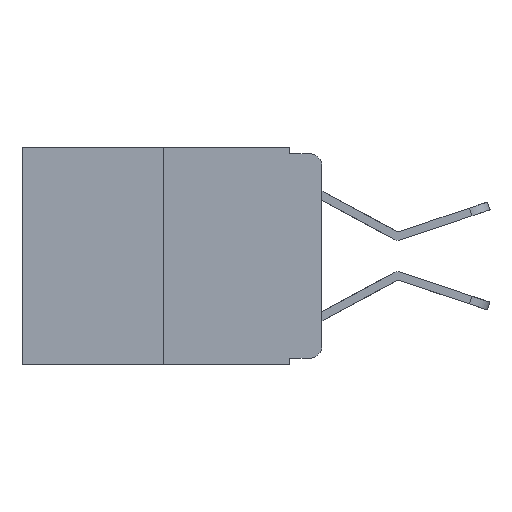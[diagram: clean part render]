
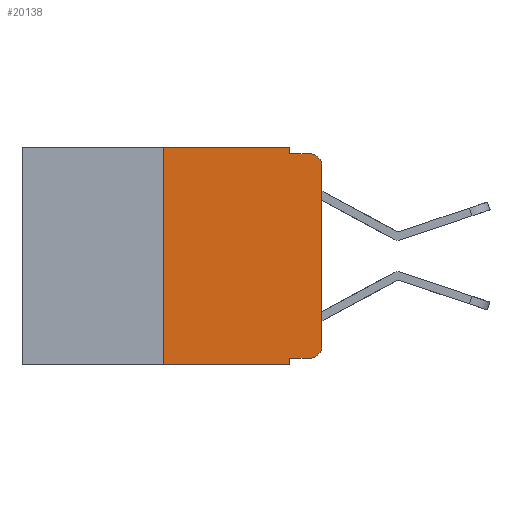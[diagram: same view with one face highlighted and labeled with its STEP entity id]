
A CAD part, left-side view. The second image highlights one B-rep face of the part: STEP entity #20138.
In plain terms, the highlighted planar face has unit normal (-1, 0, 0).
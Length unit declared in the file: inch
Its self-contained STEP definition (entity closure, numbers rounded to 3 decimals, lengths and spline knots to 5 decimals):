
#455 = ORIENTED_EDGE ( 'NONE', *, *, #19903, .F. ) ;
#567 = VERTEX_POINT ( 'NONE', #24018 ) ;
#948 = CARTESIAN_POINT ( 'NONE',  ( 0., 0.25, 0. ) ) ;
#1726 = EDGE_CURVE ( 'NONE', #22850, #15230, #16019, .T. ) ;
#1812 = ORIENTED_EDGE ( 'NONE', *, *, #18586, .F. ) ;
#2081 = DIRECTION ( 'NONE',  ( 0., -1., 0. ) ) ;
#2087 = CARTESIAN_POINT ( 'NONE',  ( 0., 0.473, -0.343 ) ) ;
#2371 = CARTESIAN_POINT ( 'NONE',  ( 0., 0.051, -0.333 ) ) ;
#2601 = CIRCLE ( 'NONE', #25285, 0.02 ) ;
#2778 = CARTESIAN_POINT ( 'NONE',  ( 0., 0.02, -0.03 ) ) ;
#3517 = VECTOR ( 'NONE', #15218, 39.37008 ) ;
#3931 = CARTESIAN_POINT ( 'NONE',  ( 0., 0.473, 0. ) ) ;
#3943 = VECTOR ( 'NONE', #12380, 39.37008 ) ;
#4050 = CARTESIAN_POINT ( 'NONE',  ( 0., 0., -0.03 ) ) ;
#4068 = DIRECTION ( 'NONE',  ( 0., 0., -1. ) ) ;
#4159 = CIRCLE ( 'NONE', #19298, 0.02 ) ;
#4498 = CARTESIAN_POINT ( 'NONE',  ( 0., 0.051, 0. ) ) ;
#4652 = VERTEX_POINT ( 'NONE', #20913 ) ;
#4718 = CARTESIAN_POINT ( 'NONE',  ( 0., 0.051, -0.01 ) ) ;
#4933 = DIRECTION ( 'NONE',  ( 0., 0., -1. ) ) ;
#5468 = CARTESIAN_POINT ( 'NONE',  ( 0., 0.02, -0.01 ) ) ;
#6043 = DIRECTION ( 'NONE',  ( 0., 0., -1. ) ) ;
#6122 = ORIENTED_EDGE ( 'NONE', *, *, #9613, .T. ) ;
#6230 = VERTEX_POINT ( 'NONE', #2371 ) ;
#7003 = VERTEX_POINT ( 'NONE', #11039 ) ;
#7270 = CARTESIAN_POINT ( 'NONE',  ( 0., 0.051, -0.01 ) ) ;
#7398 = ORIENTED_EDGE ( 'NONE', *, *, #17284, .T. ) ;
#7729 = VECTOR ( 'NONE', #18364, 39.37008 ) ;
#7857 = LINE ( 'NONE', #17208, #17907 ) ;
#8035 = CARTESIAN_POINT ( 'NONE',  ( 0., 0.02, -0.313 ) ) ;
#8045 = ORIENTED_EDGE ( 'NONE', *, *, #14597, .T. ) ;
#8287 = CARTESIAN_POINT ( 'NONE',  ( 0., 0.25, 0. ) ) ;
#8868 = LINE ( 'NONE', #18357, #19197 ) ;
#8964 = DIRECTION ( 'NONE',  ( 0., -1., 0. ) ) ;
#9008 = ORIENTED_EDGE ( 'NONE', *, *, #1726, .T. ) ;
#9306 = CARTESIAN_POINT ( 'NONE',  ( 0., 0., -0.313 ) ) ;
#9437 = LINE ( 'NONE', #15255, #25722 ) ;
#9613 = EDGE_CURVE ( 'NONE', #4652, #567, #13111, .T. ) ;
#9634 = VECTOR ( 'NONE', #4068, 39.37008 ) ;
#10115 = DIRECTION ( 'NONE',  ( 0., 0., -1. ) ) ;
#10415 = AXIS2_PLACEMENT_3D ( 'NONE', #3931, #18091, #6043 ) ;
#11039 = CARTESIAN_POINT ( 'NONE',  ( 0., 0.02, -0.333 ) ) ;
#12074 = PLANE ( 'NONE',  #10415 ) ;
#12380 = DIRECTION ( 'NONE',  ( 0., 0., 1. ) ) ;
#12820 = FACE_OUTER_BOUND ( 'NONE', #22519, .T. ) ;
#13111 = LINE ( 'NONE', #2087, #7729 ) ;
#13141 = LINE ( 'NONE', #948, #3517 ) ;
#14327 = ORIENTED_EDGE ( 'NONE', *, *, #25070, .T. ) ;
#14597 = EDGE_CURVE ( 'NONE', #7003, #22850, #4159, .T. ) ;
#15195 = DIRECTION ( 'NONE',  ( 0., 0., -1. ) ) ;
#15218 = DIRECTION ( 'NONE',  ( 0., 0., 1. ) ) ;
#15230 = VERTEX_POINT ( 'NONE', #4050 ) ;
#15255 = CARTESIAN_POINT ( 'NONE',  ( 0., 0.473, 0. ) ) ;
#16019 = LINE ( 'NONE', #22169, #3943 ) ;
#16214 = ORIENTED_EDGE ( 'NONE', *, *, #19267, .F. ) ;
#16226 = CARTESIAN_POINT ( 'NONE',  ( 0., 0.051, 0. ) ) ;
#17026 = DIRECTION ( 'NONE',  ( -1., 0., 0. ) ) ;
#17208 = CARTESIAN_POINT ( 'NONE',  ( 0., 0.051, 0. ) ) ;
#17284 = EDGE_CURVE ( 'NONE', #6230, #7003, #8868, .T. ) ;
#17777 = VERTEX_POINT ( 'NONE', #4498 ) ;
#17907 = VECTOR ( 'NONE', #15195, 39.37008 ) ;
#18091 = DIRECTION ( 'NONE',  ( 1., 0., 0. ) ) ;
#18357 = CARTESIAN_POINT ( 'NONE',  ( 0., 0.051, -0.333 ) ) ;
#18364 = DIRECTION ( 'NONE',  ( 0., -1., 0. ) ) ;
#18586 = EDGE_CURVE ( 'NONE', #6230, #567, #7857, .T. ) ;
#19197 = VECTOR ( 'NONE', #2081, 39.37008 ) ;
#19243 = DIRECTION ( 'NONE',  ( 0., -1., 0. ) ) ;
#19267 = EDGE_CURVE ( 'NONE', #20236, #17777, #9437, .T. ) ;
#19298 = AXIS2_PLACEMENT_3D ( 'NONE', #8035, #21954, #10115 ) ;
#19903 = EDGE_CURVE ( 'NONE', #4652, #20236, #13141, .T. ) ;
#20138 = ADVANCED_FACE ( 'NONE', ( #12820 ), #12074, .F. ) ;
#20204 = ORIENTED_EDGE ( 'NONE', *, *, #23780, .F. ) ;
#20236 = VERTEX_POINT ( 'NONE', #8287 ) ;
#20913 = CARTESIAN_POINT ( 'NONE',  ( 0., 0.25, -0.343 ) ) ;
#21228 = EDGE_CURVE ( 'NONE', #17777, #25181, #24097, .T. ) ;
#21954 = DIRECTION ( 'NONE',  ( -1., 0., 0. ) ) ;
#22169 = CARTESIAN_POINT ( 'NONE',  ( 0., 0., 0. ) ) ;
#22293 = VERTEX_POINT ( 'NONE', #5468 ) ;
#22519 = EDGE_LOOP ( 'NONE', ( #9008, #14327, #20204, #25329, #16214, #455, #6122, #1812, #7398, #8045 ) ) ;
#22850 = VERTEX_POINT ( 'NONE', #9306 ) ;
#23566 = VECTOR ( 'NONE', #8964, 39.37008 ) ;
#23780 = EDGE_CURVE ( 'NONE', #25181, #22293, #24175, .T. ) ;
#24018 = CARTESIAN_POINT ( 'NONE',  ( 0., 0.051, -0.343 ) ) ;
#24097 = LINE ( 'NONE', #16226, #9634 ) ;
#24175 = LINE ( 'NONE', #4718, #23566 ) ;
#25070 = EDGE_CURVE ( 'NONE', #15230, #22293, #2601, .T. ) ;
#25181 = VERTEX_POINT ( 'NONE', #7270 ) ;
#25285 = AXIS2_PLACEMENT_3D ( 'NONE', #2778, #17026, #4933 ) ;
#25329 = ORIENTED_EDGE ( 'NONE', *, *, #21228, .F. ) ;
#25722 = VECTOR ( 'NONE', #19243, 39.37008 ) ;
